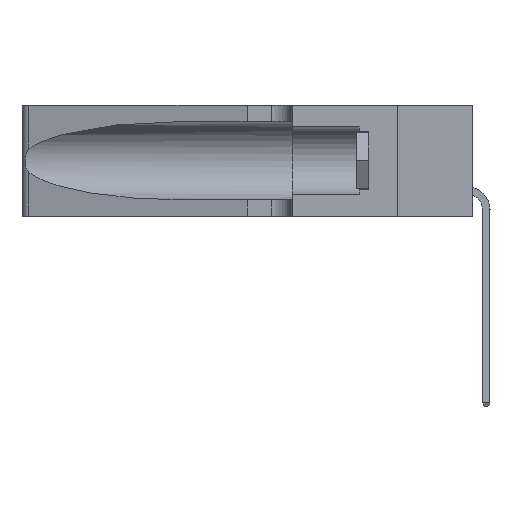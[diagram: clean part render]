
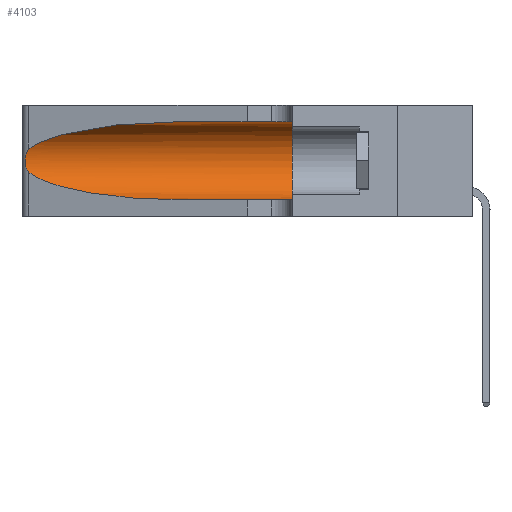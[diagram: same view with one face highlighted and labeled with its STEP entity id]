
A CAD part, left-side view. The second image highlights one B-rep face of the part: STEP entity #4103.
In plain terms, the highlighted cylindrical face has radius 3.308 mm (diameter 6.617 mm), a partial arc.
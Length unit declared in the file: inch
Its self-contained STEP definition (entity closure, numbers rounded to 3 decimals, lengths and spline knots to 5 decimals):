
#59 = CARTESIAN_POINT ( 'NONE',  ( 0.25787, 1.23484, 0.2124 ) ) ;
#91 = ORIENTED_EDGE ( 'NONE', *, *, #702, .T. ) ;
#129 = CARTESIAN_POINT ( 'NONE',  ( 0.26017, 1.23833, 0.17102 ) ) ;
#403 = CYLINDRICAL_SURFACE ( 'NONE', #2365, 0.13025 ) ;
#448 = VERTEX_POINT ( 'NONE', #857 ) ;
#702 = EDGE_CURVE ( 'NONE', #448, #4758, #9823, .T. ) ;
#857 = CARTESIAN_POINT ( 'NONE',  ( 0.25487, 1.22718, 0.22369 ) ) ;
#862 = DIRECTION ( 'NONE',  ( 0., 1., 0. ) ) ;
#1152 = VERTEX_POINT ( 'NONE', #7576 ) ;
#1161 = CARTESIAN_POINT ( 'NONE',  ( 0.1305, 1.61858, 0.185 ) ) ;
#1722 = CARTESIAN_POINT ( 'NONE',  ( 0.25789, 1.23486, 0.15765 ) ) ;
#2033 = VECTOR ( 'NONE', #2689, 39.37008 ) ;
#2354 = CARTESIAN_POINT ( 'NONE',  ( 0.1305, 0.72297, 0.05475 ) ) ;
#2365 = AXIS2_PLACEMENT_3D ( 'NONE', #1161, #2739, #18577 ) ;
#2437 = DIRECTION ( 'NONE',  ( 0., 0., 1. ) ) ;
#2689 = DIRECTION ( 'NONE',  ( 0., -1., 0. ) ) ;
#2739 = DIRECTION ( 'NONE',  ( 0., -1., 0. ) ) ;
#3223 = CARTESIAN_POINT ( 'NONE',  ( 0.25639, 1.23184, 0.21858 ) ) ;
#3918 = ORIENTED_EDGE ( 'NONE', *, *, #9601, .F. ) ;
#4103 = ADVANCED_FACE ( 'NONE', ( #17329 ), #403, .F. ) ;
#4404 = CARTESIAN_POINT ( 'NONE',  ( 0.1305, 0.72297, 0.05475 ) ) ;
#4412 = DIRECTION ( 'NONE',  ( 0., -1., 0. ) ) ;
#4537 = CARTESIAN_POINT ( 'NONE',  ( 0.25555, 1.22993, 0.14849 ) ) ;
#4601 = CARTESIAN_POINT ( 'NONE',  ( 0.2373, 1.15595, 0.08982 ) ) ;
#4758 = VERTEX_POINT ( 'NONE', #5023 ) ;
#4816 = CARTESIAN_POINT ( 'NONE',  ( 0.26018, 1.23835, 0.19895 ) ) ;
#4976 = LINE ( 'NONE', #5889, #2033 ) ;
#5023 = CARTESIAN_POINT ( 'NONE',  ( 0.25487, 1.22718, 0.14631 ) ) ;
#5092 = EDGE_CURVE ( 'NONE', #1152, #448, #8359, .T. ) ;
#5162 = AXIS2_PLACEMENT_3D ( 'NONE', #10184, #862, #2437 ) ;
#5402 = EDGE_CURVE ( 'NONE', #8392, #17557, #15077, .T. ) ;
#5889 = CARTESIAN_POINT ( 'NONE',  ( 0.1305, 1.61858, 0.31525 ) ) ;
#6055 = EDGE_LOOP ( 'NONE', ( #19220, #91, #16248, #8945, #3918, #20278 ) ) ;
#6107 = CARTESIAN_POINT ( 'NONE',  ( 0.25487, 1.22718, 0.14631 ) ) ;
#6987 = EDGE_CURVE ( 'NONE', #1152, #14844, #4976, .T. ) ;
#7576 = CARTESIAN_POINT ( 'NONE',  ( 0.1305, 0.72297, 0.31525 ) ) ;
#8152 = CARTESIAN_POINT ( 'NONE',  ( 0.1305, 0.35, 0.31525 ) ) ;
#8359 =( BOUNDED_CURVE ( )  B_SPLINE_CURVE ( 3, ( #17705, #11486, #13241, #19435 ),
 .UNSPECIFIED., .F., .F. ) 
 B_SPLINE_CURVE_WITH_KNOTS ( ( 4, 4 ),
 ( 1.5708, 2.84003 ),
 .UNSPECIFIED. ) 
 CURVE ( )  GEOMETRIC_REPRESENTATION_ITEM ( )  RATIONAL_B_SPLINE_CURVE ( ( 1., 0.87, 0.87, 1. ) ) 
 REPRESENTATION_ITEM ( '' )  );
#8392 = VERTEX_POINT ( 'NONE', #2354 ) ;
#8945 = ORIENTED_EDGE ( 'NONE', *, *, #5402, .T. ) ;
#9229 = CARTESIAN_POINT ( 'NONE',  ( 0.26075, 1.23896, 0.19203 ) ) ;
#9395 = CIRCLE ( 'NONE', #5162, 0.13025 ) ;
#9425 = CARTESIAN_POINT ( 'NONE',  ( 0.25487, 1.22718, 0.22369 ) ) ;
#9601 = EDGE_CURVE ( 'NONE', #14844, #17557, #9395, .T. ) ;
#9823 = B_SPLINE_CURVE_WITH_KNOTS ( 'NONE', 3,
 ( #9425, #11039, #3223, #59, #20159, #4816, #9229, #10767, #129, #15455, #1722, #12594, #4537, #6107 ),
 .UNSPECIFIED., .F., .F.,
 ( 4, 2, 2, 2, 2, 2, 4 ),
 ( 0., 0.00027, 0.00053, 0.00107, 0.0016, 0.00187, 0.00214 ),
 .UNSPECIFIED. ) ;
#10184 = CARTESIAN_POINT ( 'NONE',  ( 0.1305, 0.35, 0.185 ) ) ;
#10767 = CARTESIAN_POINT ( 'NONE',  ( 0.26075, 1.23896, 0.178 ) ) ;
#10870 = VECTOR ( 'NONE', #4412, 39.37008 ) ;
#11039 = CARTESIAN_POINT ( 'NONE',  ( 0.25555, 1.22994, 0.2215 ) ) ;
#11486 = CARTESIAN_POINT ( 'NONE',  ( 0.18966, 0.96281, 0.31525 ) ) ;
#12594 = CARTESIAN_POINT ( 'NONE',  ( 0.25639, 1.23186, 0.15144 ) ) ;
#13241 = CARTESIAN_POINT ( 'NONE',  ( 0.2373, 1.15595, 0.28018 ) ) ;
#13916 = CARTESIAN_POINT ( 'NONE',  ( 0.25487, 1.22718, 0.14631 ) ) ;
#14844 = VERTEX_POINT ( 'NONE', #8152 ) ;
#15077 = LINE ( 'NONE', #16876, #10870 ) ;
#15455 = CARTESIAN_POINT ( 'NONE',  ( 0.25856, 1.23593, 0.16098 ) ) ;
#15969 =( BOUNDED_CURVE ( )  B_SPLINE_CURVE ( 3, ( #13916, #4601, #19962, #4404 ),
 .UNSPECIFIED., .F., .T. ) 
 B_SPLINE_CURVE_WITH_KNOTS ( ( 4, 4 ),
 ( 3.44316, 4.71239 ),
 .UNSPECIFIED. ) 
 CURVE ( )  GEOMETRIC_REPRESENTATION_ITEM ( )  RATIONAL_B_SPLINE_CURVE ( ( 1., 0.87, 0.87, 1. ) ) 
 REPRESENTATION_ITEM ( '' )  );
#16248 = ORIENTED_EDGE ( 'NONE', *, *, #17113, .T. ) ;
#16876 = CARTESIAN_POINT ( 'NONE',  ( 0.1305, 1.61858, 0.05475 ) ) ;
#17113 = EDGE_CURVE ( 'NONE', #4758, #8392, #15969, .T. ) ;
#17329 = FACE_OUTER_BOUND ( 'NONE', #6055, .T. ) ;
#17557 = VERTEX_POINT ( 'NONE', #17704 ) ;
#17704 = CARTESIAN_POINT ( 'NONE',  ( 0.1305, 0.35, 0.05475 ) ) ;
#17705 = CARTESIAN_POINT ( 'NONE',  ( 0.1305, 0.72297, 0.31525 ) ) ;
#18577 = DIRECTION ( 'NONE',  ( 0., 0., -1. ) ) ;
#19220 = ORIENTED_EDGE ( 'NONE', *, *, #5092, .T. ) ;
#19435 = CARTESIAN_POINT ( 'NONE',  ( 0.25487, 1.22718, 0.22369 ) ) ;
#19962 = CARTESIAN_POINT ( 'NONE',  ( 0.18966, 0.96281, 0.05475 ) ) ;
#20159 = CARTESIAN_POINT ( 'NONE',  ( 0.25854, 1.2359, 0.20912 ) ) ;
#20278 = ORIENTED_EDGE ( 'NONE', *, *, #6987, .F. ) ;
